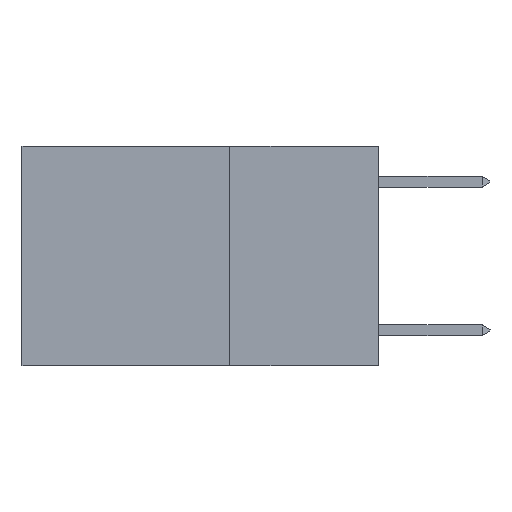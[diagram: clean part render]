
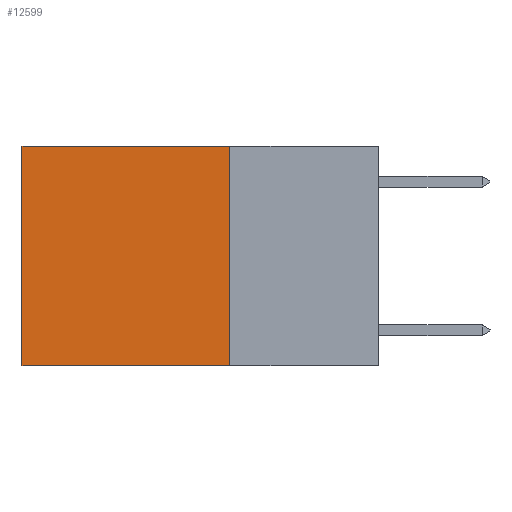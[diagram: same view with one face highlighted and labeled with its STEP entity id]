
A CAD part, left-side view. The second image highlights one B-rep face of the part: STEP entity #12599.
In plain terms, the highlighted planar face has unit normal (-1, 0, 0).
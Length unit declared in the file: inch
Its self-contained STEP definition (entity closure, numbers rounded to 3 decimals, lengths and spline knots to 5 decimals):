
#357 = LINE ( 'NONE', #17654, #17159 ) ;
#1155 = EDGE_CURVE ( 'NONE', #12359, #20126, #357, .T. ) ;
#1848 = DIRECTION ( 'NONE',  ( 1., 0., 0. ) ) ;
#2455 = EDGE_LOOP ( 'NONE', ( #12427, #15308, #11366, #5723 ) ) ;
#3284 = FACE_OUTER_BOUND ( 'NONE', #2455, .T. ) ;
#3363 = CARTESIAN_POINT ( 'NONE',  ( 0.2625, 0.25, 0. ) ) ;
#3679 = VECTOR ( 'NONE', #10259, 39.37008 ) ;
#3910 = DIRECTION ( 'NONE',  ( 0., 1., 0. ) ) ;
#4312 = VERTEX_POINT ( 'NONE', #13903 ) ;
#4578 = CARTESIAN_POINT ( 'NONE',  ( 0.2625, 0.25, 0. ) ) ;
#5497 = CARTESIAN_POINT ( 'NONE',  ( 0.2625, 0.25, -0.37 ) ) ;
#5723 = ORIENTED_EDGE ( 'NONE', *, *, #1155, .T. ) ;
#7896 = LINE ( 'NONE', #16562, #3679 ) ;
#8496 = EDGE_CURVE ( 'NONE', #4312, #12001, #17273, .T. ) ;
#9775 = DIRECTION ( 'NONE',  ( 0., 1., 0. ) ) ;
#10259 = DIRECTION ( 'NONE',  ( 0., 0., -1. ) ) ;
#11302 = PLANE ( 'NONE',  #13984 ) ;
#11366 = ORIENTED_EDGE ( 'NONE', *, *, #11676, .F. ) ;
#11676 = EDGE_CURVE ( 'NONE', #12359, #4312, #19151, .T. ) ;
#12001 = VERTEX_POINT ( 'NONE', #16310 ) ;
#12359 = VERTEX_POINT ( 'NONE', #20225 ) ;
#12427 = ORIENTED_EDGE ( 'NONE', *, *, #17861, .T. ) ;
#12599 = ADVANCED_FACE ( 'NONE', ( #3284 ), #11302, .F. ) ;
#12927 = DIRECTION ( 'NONE',  ( 0., 0., -1. ) ) ;
#13099 = VECTOR ( 'NONE', #3910, 39.37008 ) ;
#13903 = CARTESIAN_POINT ( 'NONE',  ( 0.2625, 0.25, -0.37 ) ) ;
#13984 = AXIS2_PLACEMENT_3D ( 'NONE', #3363, #1848, #12927 ) ;
#14961 = VECTOR ( 'NONE', #17213, 39.37008 ) ;
#15308 = ORIENTED_EDGE ( 'NONE', *, *, #8496, .F. ) ;
#16310 = CARTESIAN_POINT ( 'NONE',  ( 0.2625, 0.6, -0.37 ) ) ;
#16562 = CARTESIAN_POINT ( 'NONE',  ( 0.2625, 0.6, 0. ) ) ;
#17034 = CARTESIAN_POINT ( 'NONE',  ( 0.2625, 0.6, 0. ) ) ;
#17159 = VECTOR ( 'NONE', #9775, 39.37008 ) ;
#17213 = DIRECTION ( 'NONE',  ( 0., 0., -1. ) ) ;
#17273 = LINE ( 'NONE', #5497, #13099 ) ;
#17654 = CARTESIAN_POINT ( 'NONE',  ( 0.2625, 0.25, 0. ) ) ;
#17861 = EDGE_CURVE ( 'NONE', #20126, #12001, #7896, .T. ) ;
#19151 = LINE ( 'NONE', #4578, #14961 ) ;
#20126 = VERTEX_POINT ( 'NONE', #17034 ) ;
#20225 = CARTESIAN_POINT ( 'NONE',  ( 0.2625, 0.25, 0. ) ) ;
